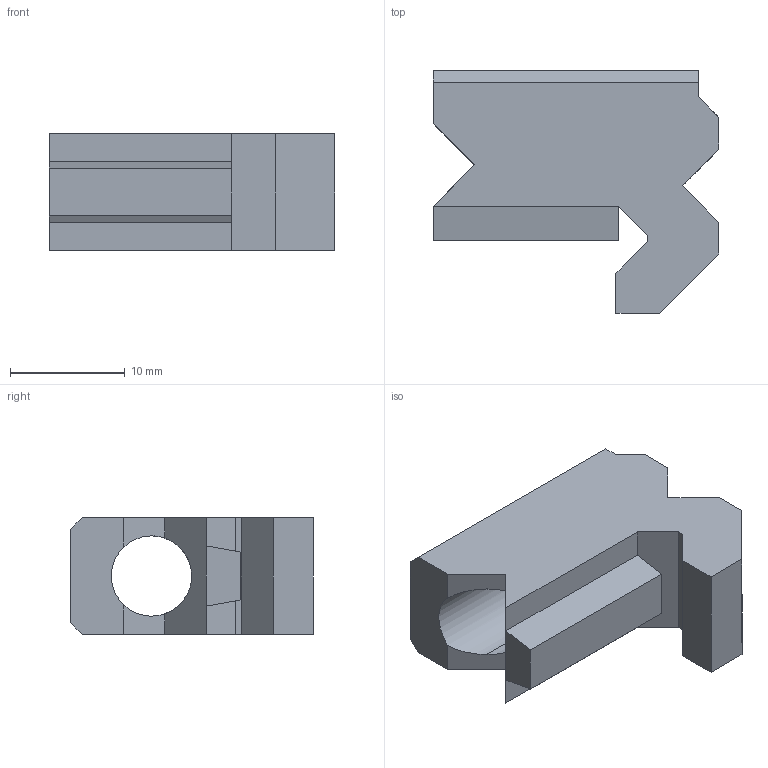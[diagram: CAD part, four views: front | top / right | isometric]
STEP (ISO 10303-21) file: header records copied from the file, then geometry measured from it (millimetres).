
FILE_DESCRIPTION (( 'STEP AP203' ), '1' );
FILE_NAME ('AF-WF-MI-PRT-002-STEP.STEP', '2020-07-21T23:49:28', ( '' ), ( '' ), 'SwSTEP 2.0', 'SolidWorks 2018', '' );
FILE_SCHEMA (( 'CONFIG_CONTROL_DESIGN' ));
Length unit declared in the file: inch
Products named in the file (1): AF-WF-MI-PRT-002-STEP
Bounding box: 24.88 x 21.12 x 10.16 mm (x, y, z)
Volume: 2668.9 mm3; surface area: 2096.6 mm2
Topology: 1 solids, 1 shells, 32 faces, 92 edges, 60 vertices
Faces by surface type: plane 30, cylinder 2
Entity records: 1110 total; most frequent: CARTESIAN_POINT 218, ORIENTED_EDGE 184, DIRECTION 150, EDGE_CURVE 92, VECTOR 78, LINE 78, VERTEX_POINT 60, AXIS2_PLACEMENT_3D 36
